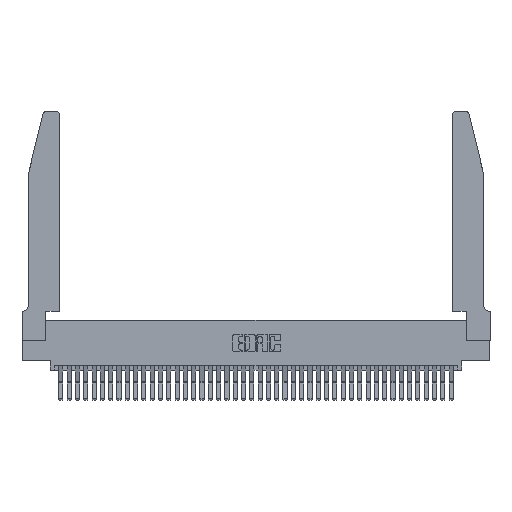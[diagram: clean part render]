
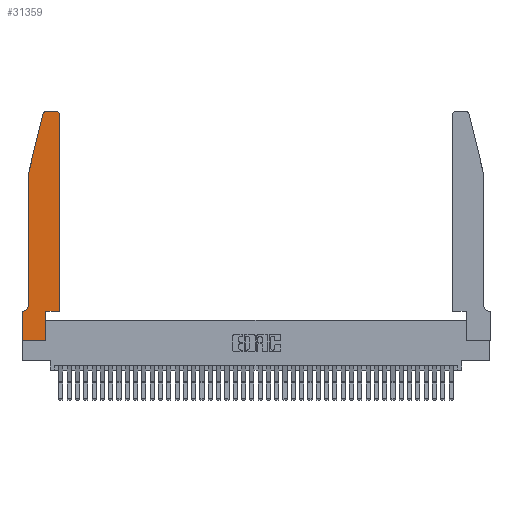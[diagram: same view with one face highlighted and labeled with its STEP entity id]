
A CAD part, top view. The second image highlights one B-rep face of the part: STEP entity #31359.
In plain terms, the highlighted planar face has unit normal (0, 0, 1).
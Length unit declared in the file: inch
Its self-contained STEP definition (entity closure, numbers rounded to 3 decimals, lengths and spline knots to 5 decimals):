
#262 = EDGE_CURVE ( 'NONE', #17246, #38532, #15494, .T. ) ;
#365 = LINE ( 'NONE', #10912, #32765 ) ;
#664 = DIRECTION ( 'NONE',  ( 1., 0., 0. ) ) ;
#709 = DIRECTION ( 'NONE',  ( -1., 0., 0. ) ) ;
#1203 = CARTESIAN_POINT ( 'NONE',  ( 0.0055, 0.35, 0.37 ) ) ;
#1245 = DIRECTION ( 'NONE',  ( -0.239, -0.971, 0. ) ) ;
#1342 = LINE ( 'NONE', #29851, #26094 ) ;
#1719 = DIRECTION ( 'NONE',  ( 0., 0., 1. ) ) ;
#2366 = VERTEX_POINT ( 'NONE', #34139 ) ;
#4877 = PLANE ( 'NONE',  #27334 ) ;
#5254 = LINE ( 'NONE', #12490, #16781 ) ;
#5300 = CARTESIAN_POINT ( 'NONE',  ( 0., 0.35, 0.37 ) ) ;
#5567 = ORIENTED_EDGE ( 'NONE', *, *, #19470, .T. ) ;
#5973 = DIRECTION ( 'NONE',  ( 1., 0., 0. ) ) ;
#6264 = CARTESIAN_POINT ( 'NONE',  ( 0.4505, 0.35, 0.37 ) ) ;
#6339 = VECTOR ( 'NONE', #5973, 39.37008 ) ;
#7208 = EDGE_CURVE ( 'NONE', #31630, #13541, #21691, .T. ) ;
#7594 = EDGE_CURVE ( 'NONE', #12357, #29466, #365, .T. ) ;
#8081 = EDGE_CURVE ( 'NONE', #29466, #31630, #35753, .T. ) ;
#9302 = ORIENTED_EDGE ( 'NONE', *, *, #31454, .T. ) ;
#10113 = EDGE_CURVE ( 'NONE', #28402, #12357, #40747, .T. ) ;
#10350 = AXIS2_PLACEMENT_3D ( 'NONE', #16197, #31907, #31781 ) ;
#10719 = DIRECTION ( 'NONE',  ( 0., 0., 1. ) ) ;
#10884 = EDGE_CURVE ( 'NONE', #24914, #17246, #21943, .T. ) ;
#10912 = CARTESIAN_POINT ( 'NONE',  ( 0.0755, 2., 0.37 ) ) ;
#11070 = ORIENTED_EDGE ( 'NONE', *, *, #8081, .T. ) ;
#11940 = VECTOR ( 'NONE', #12206, 39.37008 ) ;
#12187 = VECTOR ( 'NONE', #29483, 39.37008 ) ;
#12206 = DIRECTION ( 'NONE',  ( 1., 0., 0. ) ) ;
#12357 = VERTEX_POINT ( 'NONE', #33183 ) ;
#12463 = LINE ( 'NONE', #31529, #11940 ) ;
#12490 = CARTESIAN_POINT ( 'NONE',  ( 0., 0., 0.37 ) ) ;
#13541 = VERTEX_POINT ( 'NONE', #1203 ) ;
#13543 = VECTOR ( 'NONE', #15093, 39.37008 ) ;
#14375 = ORIENTED_EDGE ( 'NONE', *, *, #262, .T. ) ;
#15093 = DIRECTION ( 'NONE',  ( -1., 0., 0. ) ) ;
#15277 = CARTESIAN_POINT ( 'NONE',  ( 0.4505, 0.35, 0.37 ) ) ;
#15494 = LINE ( 'NONE', #15277, #23594 ) ;
#15942 = FACE_OUTER_BOUND ( 'NONE', #35919, .T. ) ;
#16197 = CARTESIAN_POINT ( 'NONE',  ( 0.0055, 0.42, 0.37 ) ) ;
#16781 = VECTOR ( 'NONE', #35472, 39.37008 ) ;
#17246 = VERTEX_POINT ( 'NONE', #6264 ) ;
#17703 = CARTESIAN_POINT ( 'NONE',  ( 0.0755, 2., 0.37 ) ) ;
#19215 = CARTESIAN_POINT ( 'NONE',  ( 0.2865, 0.35, 0.37 ) ) ;
#19470 = EDGE_CURVE ( 'NONE', #13541, #38967, #41396, .T. ) ;
#20037 = DIRECTION ( 'NONE',  ( 0., 0., 1. ) ) ;
#20876 = EDGE_CURVE ( 'NONE', #2366, #28402, #1342, .T. ) ;
#21691 = CIRCLE ( 'NONE', #10350, 0.07 ) ;
#21740 = LINE ( 'NONE', #19215, #12187 ) ;
#21943 = LINE ( 'NONE', #22753, #6339 ) ;
#22007 = AXIS2_PLACEMENT_3D ( 'NONE', #36782, #10719, #26748 ) ;
#22295 = ORIENTED_EDGE ( 'NONE', *, *, #7594, .T. ) ;
#22542 = CIRCLE ( 'NONE', #24365, 0.03 ) ;
#22753 = CARTESIAN_POINT ( 'NONE',  ( 0.4505, 0.35, 0.37 ) ) ;
#23594 = VECTOR ( 'NONE', #38183, 39.37008 ) ;
#23897 = VERTEX_POINT ( 'NONE', #32618 ) ;
#23952 = ORIENTED_EDGE ( 'NONE', *, *, #7208, .T. ) ;
#24365 = AXIS2_PLACEMENT_3D ( 'NONE', #35609, #20037, #664 ) ;
#24496 = ORIENTED_EDGE ( 'NONE', *, *, #20876, .T. ) ;
#24528 = ORIENTED_EDGE ( 'NONE', *, *, #10113, .T. ) ;
#24914 = VERTEX_POINT ( 'NONE', #37113 ) ;
#25415 = VERTEX_POINT ( 'NONE', #39484 ) ;
#26094 = VECTOR ( 'NONE', #709, 39.37008 ) ;
#26748 = DIRECTION ( 'NONE',  ( 1., 0., 0. ) ) ;
#26963 = EDGE_CURVE ( 'NONE', #38967, #25415, #5254, .T. ) ;
#27334 = AXIS2_PLACEMENT_3D ( 'NONE', #5300, #1719, #30530 ) ;
#28402 = VERTEX_POINT ( 'NONE', #37048 ) ;
#28986 = EDGE_CURVE ( 'NONE', #23897, #24914, #21740, .T. ) ;
#29466 = VERTEX_POINT ( 'NONE', #35494 ) ;
#29483 = DIRECTION ( 'NONE',  ( 0., 1., 0. ) ) ;
#29851 = CARTESIAN_POINT ( 'NONE',  ( 0.2605, 2.75, 0.37 ) ) ;
#30530 = DIRECTION ( 'NONE',  ( 1., 0., 0. ) ) ;
#30787 = CARTESIAN_POINT ( 'NONE',  ( 0., 0.35, 0.37 ) ) ;
#31009 = ORIENTED_EDGE ( 'NONE', *, *, #26963, .T. ) ;
#31159 = EDGE_CURVE ( 'NONE', #38532, #2366, #22542, .T. ) ;
#31359 = ADVANCED_FACE ( 'NONE', ( #15942 ), #4877, .T. ) ;
#31454 = EDGE_CURVE ( 'NONE', #25415, #23897, #12463, .T. ) ;
#31529 = CARTESIAN_POINT ( 'NONE',  ( 0., 0., 0.37 ) ) ;
#31630 = VERTEX_POINT ( 'NONE', #35548 ) ;
#31781 = DIRECTION ( 'NONE',  ( -1., 0., 0. ) ) ;
#31907 = DIRECTION ( 'NONE',  ( 0., 0., -1. ) ) ;
#32618 = CARTESIAN_POINT ( 'NONE',  ( 0.2865, 0., 0.37 ) ) ;
#32712 = ORIENTED_EDGE ( 'NONE', *, *, #10884, .T. ) ;
#32728 = VECTOR ( 'NONE', #34272, 39.37008 ) ;
#32765 = VECTOR ( 'NONE', #1245, 39.37008 ) ;
#33183 = CARTESIAN_POINT ( 'NONE',  ( 0.25487, 2.72718, 0.37 ) ) ;
#34139 = CARTESIAN_POINT ( 'NONE',  ( 0.4205, 2.75, 0.37 ) ) ;
#34186 = CARTESIAN_POINT ( 'NONE',  ( 0.0755, 0.35, 0.37 ) ) ;
#34272 = DIRECTION ( 'NONE',  ( 0., -1., 0. ) ) ;
#35380 = ORIENTED_EDGE ( 'NONE', *, *, #31159, .T. ) ;
#35472 = DIRECTION ( 'NONE',  ( 0., -1., 0. ) ) ;
#35494 = CARTESIAN_POINT ( 'NONE',  ( 0.0755, 2., 0.37 ) ) ;
#35548 = CARTESIAN_POINT ( 'NONE',  ( 0.0755, 0.42, 0.37 ) ) ;
#35609 = CARTESIAN_POINT ( 'NONE',  ( 0.4205, 2.72, 0.37 ) ) ;
#35753 = LINE ( 'NONE', #17703, #32728 ) ;
#35919 = EDGE_LOOP ( 'NONE', ( #24496, #24528, #22295, #11070, #23952, #5567, #31009, #9302, #38751, #32712, #14375, #35380 ) ) ;
#36782 = CARTESIAN_POINT ( 'NONE',  ( 0.284, 2.72, 0.37 ) ) ;
#37048 = CARTESIAN_POINT ( 'NONE',  ( 0.284, 2.75, 0.37 ) ) ;
#37113 = CARTESIAN_POINT ( 'NONE',  ( 0.2865, 0.35, 0.37 ) ) ;
#38183 = DIRECTION ( 'NONE',  ( 0., 1., 0. ) ) ;
#38465 = CARTESIAN_POINT ( 'NONE',  ( 0.4505, 2.72, 0.37 ) ) ;
#38532 = VERTEX_POINT ( 'NONE', #38465 ) ;
#38751 = ORIENTED_EDGE ( 'NONE', *, *, #28986, .T. ) ;
#38967 = VERTEX_POINT ( 'NONE', #30787 ) ;
#39484 = CARTESIAN_POINT ( 'NONE',  ( 0., 0., 0.37 ) ) ;
#40747 = CIRCLE ( 'NONE', #22007, 0.03 ) ;
#41396 = LINE ( 'NONE', #34186, #13543 ) ;
